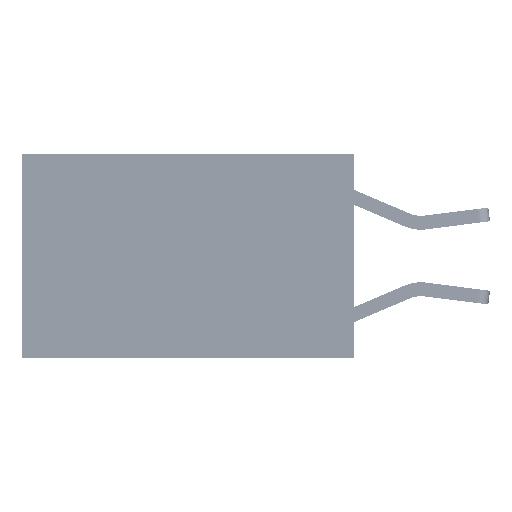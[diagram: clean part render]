
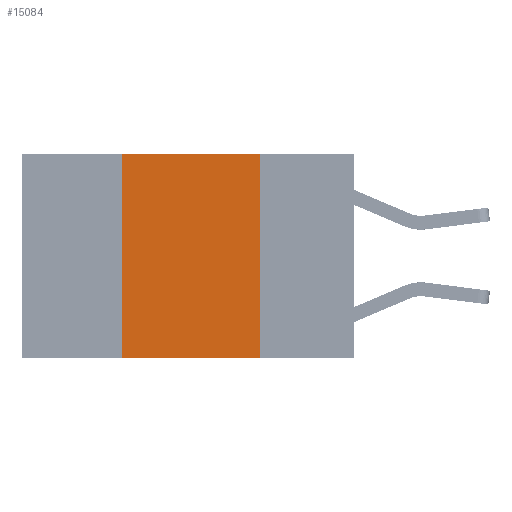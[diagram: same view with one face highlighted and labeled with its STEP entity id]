
A CAD part, left-side view. The second image highlights one B-rep face of the part: STEP entity #15084.
In plain terms, the highlighted planar face has unit normal (-1, 0, 0).
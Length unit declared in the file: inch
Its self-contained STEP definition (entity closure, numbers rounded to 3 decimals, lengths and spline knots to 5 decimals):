
#1006 = LINE ( 'NONE', #2986, #12708 ) ;
#2487 = VERTEX_POINT ( 'NONE', #13184 ) ;
#2986 = CARTESIAN_POINT ( 'NONE',  ( 0., 0.42, 0. ) ) ;
#4698 = DIRECTION ( 'NONE',  ( 0., 0., -1. ) ) ;
#4823 = CARTESIAN_POINT ( 'NONE',  ( 0., 0.17, -0.37 ) ) ;
#5328 = EDGE_LOOP ( 'NONE', ( #20739, #28785, #10214, #14921 ) ) ;
#6019 = VECTOR ( 'NONE', #21437, 39.37008 ) ;
#6186 = VERTEX_POINT ( 'NONE', #28599 ) ;
#6233 = EDGE_CURVE ( 'NONE', #18203, #7002, #9652, .T. ) ;
#7002 = VERTEX_POINT ( 'NONE', #4823 ) ;
#8990 = LINE ( 'NONE', #9146, #13844 ) ;
#9146 = CARTESIAN_POINT ( 'NONE',  ( 0., 0.6, 0. ) ) ;
#9280 = PLANE ( 'NONE',  #17432 ) ;
#9443 = FACE_OUTER_BOUND ( 'NONE', #5328, .T. ) ;
#9607 = DIRECTION ( 'NONE',  ( 1., 0., 0. ) ) ;
#9652 = LINE ( 'NONE', #12274, #25558 ) ;
#10214 = ORIENTED_EDGE ( 'NONE', *, *, #30581, .F. ) ;
#10637 = CARTESIAN_POINT ( 'NONE',  ( 0., 0.17, 0. ) ) ;
#12274 = CARTESIAN_POINT ( 'NONE',  ( 0., 0.17, 0. ) ) ;
#12708 = VECTOR ( 'NONE', #20888, 39.37008 ) ;
#13184 = CARTESIAN_POINT ( 'NONE',  ( 0., 0.42, 0. ) ) ;
#13844 = VECTOR ( 'NONE', #24464, 39.37008 ) ;
#14921 = ORIENTED_EDGE ( 'NONE', *, *, #23576, .T. ) ;
#15084 = ADVANCED_FACE ( 'NONE', ( #9443 ), #9280, .F. ) ;
#16166 = CARTESIAN_POINT ( 'NONE',  ( 0., 0.6, -0.37 ) ) ;
#17042 = DIRECTION ( 'NONE',  ( 0., 0., -1. ) ) ;
#17432 = AXIS2_PLACEMENT_3D ( 'NONE', #19308, #9607, #4698 ) ;
#18203 = VERTEX_POINT ( 'NONE', #10637 ) ;
#19308 = CARTESIAN_POINT ( 'NONE',  ( 0., 0.6, 0. ) ) ;
#20739 = ORIENTED_EDGE ( 'NONE', *, *, #6233, .F. ) ;
#20888 = DIRECTION ( 'NONE',  ( 0., 0., 1. ) ) ;
#21350 = EDGE_CURVE ( 'NONE', #2487, #18203, #8990, .T. ) ;
#21437 = DIRECTION ( 'NONE',  ( 0., -1., 0. ) ) ;
#23576 = EDGE_CURVE ( 'NONE', #6186, #7002, #26532, .T. ) ;
#24464 = DIRECTION ( 'NONE',  ( 0., -1., 0. ) ) ;
#25558 = VECTOR ( 'NONE', #17042, 39.37008 ) ;
#26532 = LINE ( 'NONE', #16166, #6019 ) ;
#28599 = CARTESIAN_POINT ( 'NONE',  ( 0., 0.42, -0.37 ) ) ;
#28785 = ORIENTED_EDGE ( 'NONE', *, *, #21350, .F. ) ;
#30581 = EDGE_CURVE ( 'NONE', #6186, #2487, #1006, .T. ) ;
